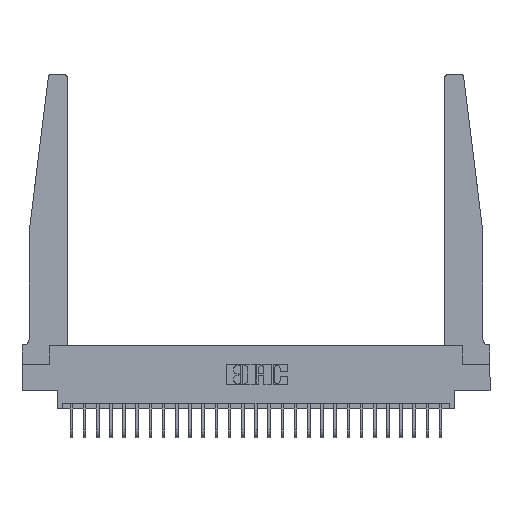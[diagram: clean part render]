
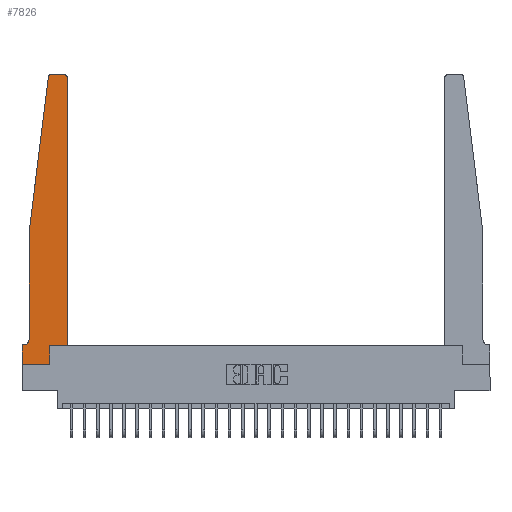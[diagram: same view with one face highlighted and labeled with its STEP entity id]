
A CAD part, top view. The second image highlights one B-rep face of the part: STEP entity #7826.
In plain terms, the highlighted planar face has unit normal (0, 0, 1).
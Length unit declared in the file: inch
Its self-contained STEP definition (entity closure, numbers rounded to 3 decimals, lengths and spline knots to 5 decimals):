
#684 = CARTESIAN_POINT ( 'NONE',  ( 0., 0., 0.37 ) ) ;
#823 = VERTEX_POINT ( 'NONE', #9347 ) ;
#1281 = CARTESIAN_POINT ( 'NONE',  ( 0.2605, 0.18, 0.37 ) ) ;
#1354 = EDGE_CURVE ( 'NONE', #21956, #6658, #3789, .T. ) ;
#2241 = ORIENTED_EDGE ( 'NONE', *, *, #25631, .T. ) ;
#2329 = ORIENTED_EDGE ( 'NONE', *, *, #7018, .T. ) ;
#2636 = VERTEX_POINT ( 'NONE', #26915 ) ;
#3065 = CIRCLE ( 'NONE', #6657, 0.03 ) ;
#3418 = DIRECTION ( 'NONE',  ( 1., 0., 0. ) ) ;
#3589 = LINE ( 'NONE', #5836, #15069 ) ;
#3695 = DIRECTION ( 'NONE',  ( 1., 0., 0. ) ) ;
#3789 = LINE ( 'NONE', #25589, #11053 ) ;
#3879 = LINE ( 'NONE', #22876, #9657 ) ;
#4038 = ORIENTED_EDGE ( 'NONE', *, *, #17803, .T. ) ;
#4219 = DIRECTION ( 'NONE',  ( 1., 0., 0. ) ) ;
#4609 = CARTESIAN_POINT ( 'NONE',  ( 0.25, 2.75, 0.37 ) ) ;
#4630 = VERTEX_POINT ( 'NONE', #11106 ) ;
#5836 = CARTESIAN_POINT ( 'NONE',  ( 0.065, 0.1875, 0.37 ) ) ;
#6083 = VECTOR ( 'NONE', #24192, 39.37008 ) ;
#6657 = AXIS2_PLACEMENT_3D ( 'NONE', #14688, #14115, #3418 ) ;
#6658 = VERTEX_POINT ( 'NONE', #12831 ) ;
#6935 = VERTEX_POINT ( 'NONE', #26583 ) ;
#7018 = EDGE_CURVE ( 'NONE', #12836, #4630, #15277, .T. ) ;
#7320 = CARTESIAN_POINT ( 'NONE',  ( 0.015, 0.2375, 0.37 ) ) ;
#7705 = LINE ( 'NONE', #16301, #17431 ) ;
#7826 = ADVANCED_FACE ( 'NONE', ( #27179 ), #7922, .T. ) ;
#7922 = PLANE ( 'NONE',  #26562 ) ;
#8021 = ORIENTED_EDGE ( 'NONE', *, *, #17652, .T. ) ;
#8093 = ORIENTED_EDGE ( 'NONE', *, *, #1354, .T. ) ;
#8096 = CARTESIAN_POINT ( 'NONE',  ( 0.395, 2.72, 0.37 ) ) ;
#8235 = DIRECTION ( 'NONE',  ( 0., 1., 0. ) ) ;
#9347 = CARTESIAN_POINT ( 'NONE',  ( 0.425, 2.72, 0.37 ) ) ;
#9547 = LINE ( 'NONE', #18148, #6083 ) ;
#9657 = VECTOR ( 'NONE', #10211, 39.37008 ) ;
#9760 = ORIENTED_EDGE ( 'NONE', *, *, #22641, .T. ) ;
#9896 = CARTESIAN_POINT ( 'NONE',  ( 0.24675, 2.72367, 0.37 ) ) ;
#9977 = EDGE_CURVE ( 'NONE', #6935, #16279, #17442, .T. ) ;
#10027 = ORIENTED_EDGE ( 'NONE', *, *, #19198, .T. ) ;
#10107 = CARTESIAN_POINT ( 'NONE',  ( 0.065, 0.2375, 0.37 ) ) ;
#10211 = DIRECTION ( 'NONE',  ( 0., -1., 0. ) ) ;
#10219 = DIRECTION ( 'NONE',  ( -0.122, -0.992, 0. ) ) ;
#11053 = VECTOR ( 'NONE', #18994, 39.37008 ) ;
#11101 = DIRECTION ( 'NONE',  ( -1., 0., 0. ) ) ;
#11106 = CARTESIAN_POINT ( 'NONE',  ( 0.015, 0.1875, 0.37 ) ) ;
#11275 = VECTOR ( 'NONE', #8235, 39.37008 ) ;
#11537 = CARTESIAN_POINT ( 'NONE',  ( 0.065, 1.25, 0.37 ) ) ;
#12082 = CIRCLE ( 'NONE', #20166, 0.03 ) ;
#12226 = EDGE_LOOP ( 'NONE', ( #13489, #18654, #9760, #4038, #2329, #14718, #17417, #8093, #10027, #8021, #17145, #2241 ) ) ;
#12610 = CARTESIAN_POINT ( 'NONE',  ( 0.425, 0.18, 0.37 ) ) ;
#12686 = LINE ( 'NONE', #23490, #16860 ) ;
#12727 = VERTEX_POINT ( 'NONE', #11537 ) ;
#12831 = CARTESIAN_POINT ( 'NONE',  ( 0.2605, 0., 0.37 ) ) ;
#12836 = VERTEX_POINT ( 'NONE', #10107 ) ;
#12889 = LINE ( 'NONE', #12610, #11275 ) ;
#13489 = ORIENTED_EDGE ( 'NONE', *, *, #9977, .T. ) ;
#13706 = EDGE_CURVE ( 'NONE', #4630, #2636, #3589, .T. ) ;
#14070 = DIRECTION ( 'NONE',  ( 0., 0., -1. ) ) ;
#14115 = DIRECTION ( 'NONE',  ( 0., 0., 1. ) ) ;
#14384 = LINE ( 'NONE', #1281, #19997 ) ;
#14688 = CARTESIAN_POINT ( 'NONE',  ( 0.27653, 2.72, 0.37 ) ) ;
#14718 = ORIENTED_EDGE ( 'NONE', *, *, #13706, .T. ) ;
#14849 = DIRECTION ( 'NONE',  ( -1., 0., 0. ) ) ;
#15069 = VECTOR ( 'NONE', #14849, 39.37008 ) ;
#15277 = CIRCLE ( 'NONE', #18849, 0.05 ) ;
#15346 = CARTESIAN_POINT ( 'NONE',  ( 0.425, 0.18, 0.37 ) ) ;
#15653 = VERTEX_POINT ( 'NONE', #9896 ) ;
#16279 = VERTEX_POINT ( 'NONE', #23906 ) ;
#16301 = CARTESIAN_POINT ( 'NONE',  ( 0.065, 1.25, 0.37 ) ) ;
#16355 = DIRECTION ( 'NONE',  ( 0., 1., 0. ) ) ;
#16554 = DIRECTION ( 'NONE',  ( 0., 0., 1. ) ) ;
#16860 = VECTOR ( 'NONE', #4219, 39.37008 ) ;
#17145 = ORIENTED_EDGE ( 'NONE', *, *, #18549, .T. ) ;
#17417 = ORIENTED_EDGE ( 'NONE', *, *, #19669, .T. ) ;
#17431 = VECTOR ( 'NONE', #10219, 39.37008 ) ;
#17442 = LINE ( 'NONE', #4609, #19113 ) ;
#17652 = EDGE_CURVE ( 'NONE', #19587, #23811, #12686, .T. ) ;
#17803 = EDGE_CURVE ( 'NONE', #12727, #12836, #9547, .T. ) ;
#18148 = CARTESIAN_POINT ( 'NONE',  ( 0.065, 1.25, 0.37 ) ) ;
#18549 = EDGE_CURVE ( 'NONE', #23811, #823, #12889, .T. ) ;
#18654 = ORIENTED_EDGE ( 'NONE', *, *, #23185, .T. ) ;
#18849 = AXIS2_PLACEMENT_3D ( 'NONE', #7320, #14070, #22497 ) ;
#18994 = DIRECTION ( 'NONE',  ( 1., 0., 0. ) ) ;
#19113 = VECTOR ( 'NONE', #11101, 39.37008 ) ;
#19198 = EDGE_CURVE ( 'NONE', #6658, #19587, #14384, .T. ) ;
#19587 = VERTEX_POINT ( 'NONE', #26396 ) ;
#19669 = EDGE_CURVE ( 'NONE', #2636, #21956, #3879, .T. ) ;
#19997 = VECTOR ( 'NONE', #16355, 39.37008 ) ;
#20166 = AXIS2_PLACEMENT_3D ( 'NONE', #8096, #16554, #26808 ) ;
#21956 = VERTEX_POINT ( 'NONE', #684 ) ;
#22497 = DIRECTION ( 'NONE',  ( -1., 0., 0. ) ) ;
#22641 = EDGE_CURVE ( 'NONE', #15653, #12727, #7705, .T. ) ;
#22876 = CARTESIAN_POINT ( 'NONE',  ( 0., 0., 0.37 ) ) ;
#22960 = DIRECTION ( 'NONE',  ( 0., 0., 1. ) ) ;
#23185 = EDGE_CURVE ( 'NONE', #16279, #15653, #3065, .T. ) ;
#23490 = CARTESIAN_POINT ( 'NONE',  ( 0.425, 0.18, 0.37 ) ) ;
#23811 = VERTEX_POINT ( 'NONE', #15346 ) ;
#23906 = CARTESIAN_POINT ( 'NONE',  ( 0.27653, 2.75, 0.37 ) ) ;
#24192 = DIRECTION ( 'NONE',  ( 0., -1., 0. ) ) ;
#25079 = CARTESIAN_POINT ( 'NONE',  ( 0., 0.1875, 0.37 ) ) ;
#25589 = CARTESIAN_POINT ( 'NONE',  ( 0., 0., 0.37 ) ) ;
#25631 = EDGE_CURVE ( 'NONE', #823, #6935, #12082, .T. ) ;
#26396 = CARTESIAN_POINT ( 'NONE',  ( 0.2605, 0.18, 0.37 ) ) ;
#26562 = AXIS2_PLACEMENT_3D ( 'NONE', #25079, #22960, #3695 ) ;
#26583 = CARTESIAN_POINT ( 'NONE',  ( 0.395, 2.75, 0.37 ) ) ;
#26808 = DIRECTION ( 'NONE',  ( 1., 0., 0. ) ) ;
#26915 = CARTESIAN_POINT ( 'NONE',  ( 0., 0.1875, 0.37 ) ) ;
#27179 = FACE_OUTER_BOUND ( 'NONE', #12226, .T. ) ;
